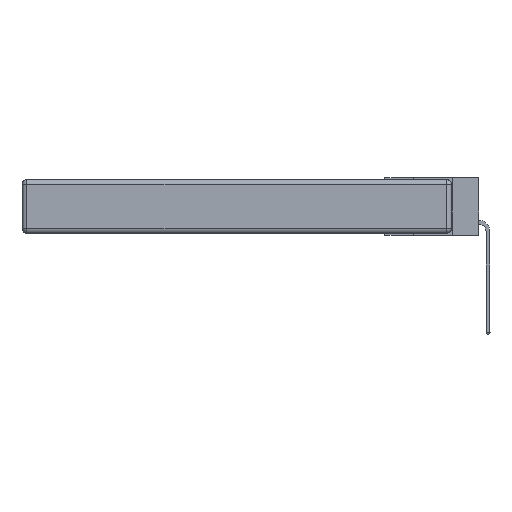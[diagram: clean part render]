
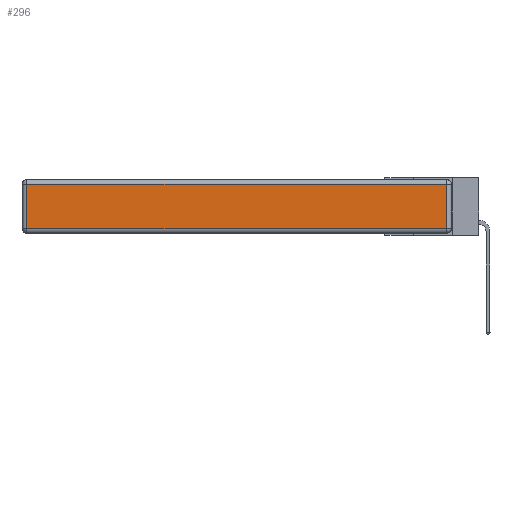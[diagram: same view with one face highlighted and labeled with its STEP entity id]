
A CAD part, left-side view. The second image highlights one B-rep face of the part: STEP entity #296.
In plain terms, the highlighted planar face has unit normal (-1, 0, 0).
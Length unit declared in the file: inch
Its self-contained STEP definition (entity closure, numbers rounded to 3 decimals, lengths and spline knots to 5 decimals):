
#296 = ADVANCED_FACE ( 'NONE', ( #6590 ), #10646, .T. ) ;
#1777 = VECTOR ( 'NONE', #2243, 39.37008 ) ;
#2243 = DIRECTION ( 'NONE',  ( 0., 0., 1. ) ) ;
#2369 = VERTEX_POINT ( 'NONE', #11313 ) ;
#3363 = LINE ( 'NONE', #18678, #19832 ) ;
#3374 = CARTESIAN_POINT ( 'NONE',  ( 0., 2.72, -0.03 ) ) ;
#4083 = DIRECTION ( 'NONE',  ( 0., 0., 1. ) ) ;
#6288 = ORIENTED_EDGE ( 'NONE', *, *, #16202, .T. ) ;
#6516 = DIRECTION ( 'NONE',  ( 0., 1., 0. ) ) ;
#6590 = FACE_OUTER_BOUND ( 'NONE', #14108, .T. ) ;
#7450 = LINE ( 'NONE', #15457, #1777 ) ;
#8861 = CARTESIAN_POINT ( 'NONE',  ( 0., 0., -0.313 ) ) ;
#8904 = VERTEX_POINT ( 'NONE', #13002 ) ;
#9605 = AXIS2_PLACEMENT_3D ( 'NONE', #17109, #13941, #4083 ) ;
#10521 = ORIENTED_EDGE ( 'NONE', *, *, #12451, .T. ) ;
#10646 = PLANE ( 'NONE',  #9605 ) ;
#10912 = DIRECTION ( 'NONE',  ( 0., 0., -1. ) ) ;
#11313 = CARTESIAN_POINT ( 'NONE',  ( 0., 0.03, -0.03 ) ) ;
#12409 = LINE ( 'NONE', #8861, #16535 ) ;
#12451 = EDGE_CURVE ( 'NONE', #8904, #2369, #7450, .T. ) ;
#13002 = CARTESIAN_POINT ( 'NONE',  ( 0., 0.03, -0.313 ) ) ;
#13388 = VERTEX_POINT ( 'NONE', #13772 ) ;
#13772 = CARTESIAN_POINT ( 'NONE',  ( 0., 2.72, -0.313 ) ) ;
#13941 = DIRECTION ( 'NONE',  ( -1., 0., 0. ) ) ;
#14108 = EDGE_LOOP ( 'NONE', ( #14997, #10521, #16758, #6288 ) ) ;
#14997 = ORIENTED_EDGE ( 'NONE', *, *, #15556, .T. ) ;
#15032 = VERTEX_POINT ( 'NONE', #3374 ) ;
#15457 = CARTESIAN_POINT ( 'NONE',  ( 0., 0.03, -0.343 ) ) ;
#15556 = EDGE_CURVE ( 'NONE', #13388, #8904, #12409, .T. ) ;
#15886 = VECTOR ( 'NONE', #6516, 39.37008 ) ;
#16202 = EDGE_CURVE ( 'NONE', #15032, #13388, #3363, .T. ) ;
#16535 = VECTOR ( 'NONE', #18910, 39.37008 ) ;
#16669 = LINE ( 'NONE', #21171, #15886 ) ;
#16758 = ORIENTED_EDGE ( 'NONE', *, *, #21135, .T. ) ;
#17109 = CARTESIAN_POINT ( 'NONE',  ( 0., 0., -0.343 ) ) ;
#18678 = CARTESIAN_POINT ( 'NONE',  ( 0., 2.72, -0.343 ) ) ;
#18910 = DIRECTION ( 'NONE',  ( 0., -1., 0. ) ) ;
#19832 = VECTOR ( 'NONE', #10912, 39.37008 ) ;
#21135 = EDGE_CURVE ( 'NONE', #2369, #15032, #16669, .T. ) ;
#21171 = CARTESIAN_POINT ( 'NONE',  ( 0., 2.75, -0.03 ) ) ;
